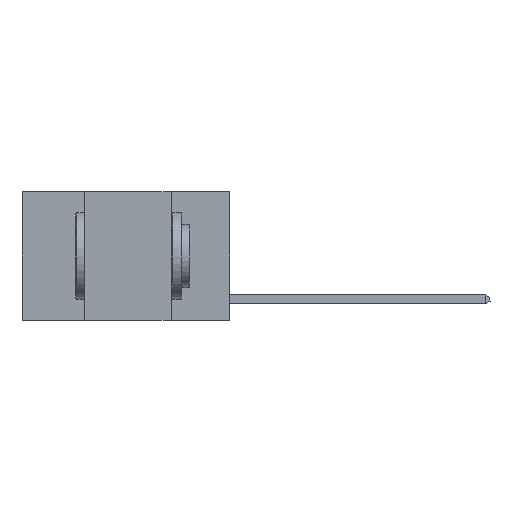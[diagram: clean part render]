
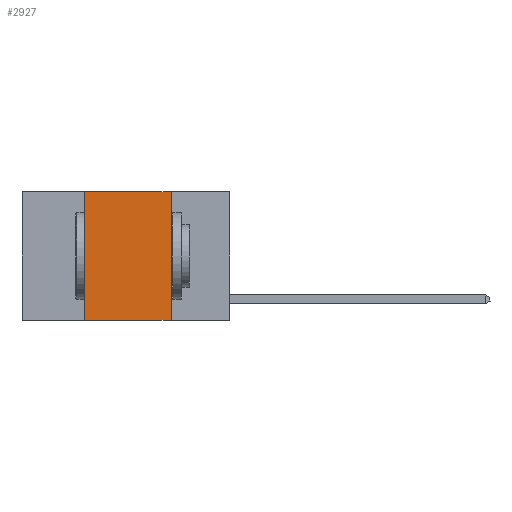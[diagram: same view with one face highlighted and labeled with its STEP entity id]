
A CAD part, left-side view. The second image highlights one B-rep face of the part: STEP entity #2927.
In plain terms, the highlighted planar face has unit normal (-1, 0, 0).
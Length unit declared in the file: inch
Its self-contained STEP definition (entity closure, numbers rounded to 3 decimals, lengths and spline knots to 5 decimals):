
#785 = CARTESIAN_POINT ( 'NONE',  ( 0., 0.6, 0. ) ) ;
#1209 = PLANE ( 'NONE',  #5064 ) ;
#1377 = VERTEX_POINT ( 'NONE', #10306 ) ;
#1444 = LINE ( 'NONE', #8713, #2883 ) ;
#1503 = DIRECTION ( 'NONE',  ( 0., 0., 1. ) ) ;
#1834 = CARTESIAN_POINT ( 'NONE',  ( 0., 0.17, -0.37 ) ) ;
#1842 = ORIENTED_EDGE ( 'NONE', *, *, #7582, .T. ) ;
#2039 = CARTESIAN_POINT ( 'NONE',  ( 0., 0.17, 0. ) ) ;
#2052 = VERTEX_POINT ( 'NONE', #1834 ) ;
#2157 = DIRECTION ( 'NONE',  ( 1., 0., 0. ) ) ;
#2530 = VERTEX_POINT ( 'NONE', #11157 ) ;
#2562 = CARTESIAN_POINT ( 'NONE',  ( 0., 0.42, -0.37 ) ) ;
#2883 = VECTOR ( 'NONE', #1503, 39.37008 ) ;
#2927 = ADVANCED_FACE ( 'NONE', ( #4687 ), #1209, .F. ) ;
#3175 = DIRECTION ( 'NONE',  ( 0., -1., 0. ) ) ;
#3792 = DIRECTION ( 'NONE',  ( 0., 0., -1. ) ) ;
#4223 = ORIENTED_EDGE ( 'NONE', *, *, #10739, .F. ) ;
#4687 = FACE_OUTER_BOUND ( 'NONE', #10790, .T. ) ;
#4944 = LINE ( 'NONE', #2039, #10149 ) ;
#5064 = AXIS2_PLACEMENT_3D ( 'NONE', #8360, #2157, #3792 ) ;
#5288 = VERTEX_POINT ( 'NONE', #2562 ) ;
#5689 = ORIENTED_EDGE ( 'NONE', *, *, #11264, .F. ) ;
#7026 = CARTESIAN_POINT ( 'NONE',  ( 0., 0.6, -0.37 ) ) ;
#7198 = LINE ( 'NONE', #785, #10358 ) ;
#7582 = EDGE_CURVE ( 'NONE', #5288, #2052, #7804, .T. ) ;
#7804 = LINE ( 'NONE', #7026, #9417 ) ;
#8360 = CARTESIAN_POINT ( 'NONE',  ( 0., 0.6, 0. ) ) ;
#8713 = CARTESIAN_POINT ( 'NONE',  ( 0., 0.42, 0. ) ) ;
#9041 = DIRECTION ( 'NONE',  ( 0., -1., 0. ) ) ;
#9417 = VECTOR ( 'NONE', #3175, 39.37008 ) ;
#10149 = VECTOR ( 'NONE', #10270, 39.37008 ) ;
#10175 = ORIENTED_EDGE ( 'NONE', *, *, #10496, .F. ) ;
#10270 = DIRECTION ( 'NONE',  ( 0., 0., -1. ) ) ;
#10306 = CARTESIAN_POINT ( 'NONE',  ( 0., 0.42, 0. ) ) ;
#10358 = VECTOR ( 'NONE', #9041, 39.37008 ) ;
#10496 = EDGE_CURVE ( 'NONE', #2530, #2052, #4944, .T. ) ;
#10739 = EDGE_CURVE ( 'NONE', #5288, #1377, #1444, .T. ) ;
#10790 = EDGE_LOOP ( 'NONE', ( #10175, #5689, #4223, #1842 ) ) ;
#11157 = CARTESIAN_POINT ( 'NONE',  ( 0., 0.17, 0. ) ) ;
#11264 = EDGE_CURVE ( 'NONE', #1377, #2530, #7198, .T. ) ;
